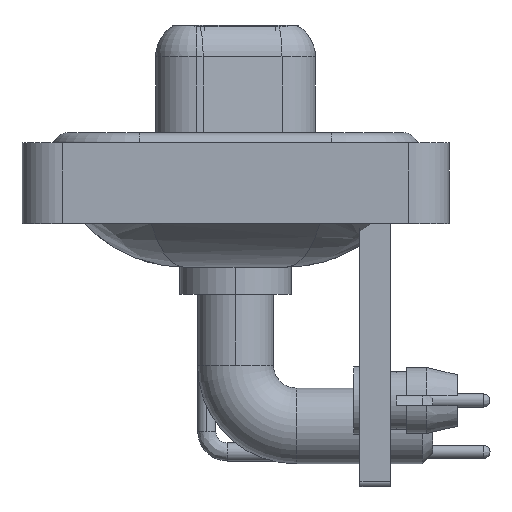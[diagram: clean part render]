
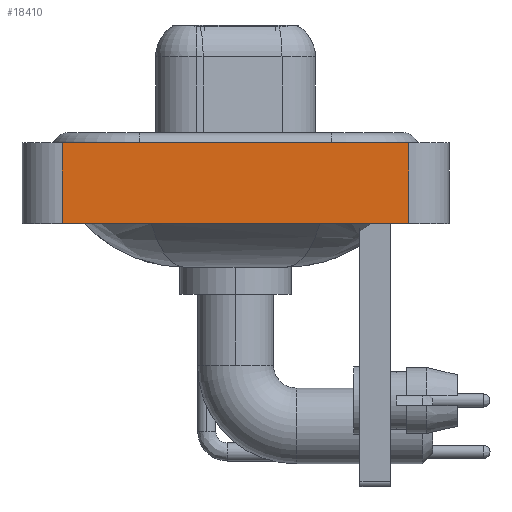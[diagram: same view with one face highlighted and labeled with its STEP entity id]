
A CAD part, left-side view. The second image highlights one B-rep face of the part: STEP entity #18410.
In plain terms, the highlighted planar face has unit normal (-1, 0, 0).
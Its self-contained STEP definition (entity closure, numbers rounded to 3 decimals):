
#1458 = EDGE_CURVE ( 'NONE', #16664, #22199, #5912, .T. ) ;
#3110 = CARTESIAN_POINT ( 'NONE',  ( -7.35, 8.55, -3.6 ) ) ;
#3141 = CARTESIAN_POINT ( 'NONE',  ( -7.35, 8.55, 0.4 ) ) ;
#4253 = CARTESIAN_POINT ( 'NONE',  ( -7.35, -8.55, -3.6 ) ) ;
#4636 = DIRECTION ( 'NONE',  ( 0., 0., 1. ) ) ;
#4999 = ORIENTED_EDGE ( 'NONE', *, *, #1458, .T. ) ;
#5130 = CARTESIAN_POINT ( 'NONE',  ( -7.35, -8.55, -3.6 ) ) ;
#5541 = VECTOR ( 'NONE', #20622, 1000. ) ;
#5754 = CARTESIAN_POINT ( 'NONE',  ( -7.35, -8.55, -3.6 ) ) ;
#5912 = LINE ( 'NONE', #4253, #5541 ) ;
#7413 = ORIENTED_EDGE ( 'NONE', *, *, #11222, .T. ) ;
#7747 = CARTESIAN_POINT ( 'NONE',  ( -7.35, -8.55, 0.4 ) ) ;
#8289 = VERTEX_POINT ( 'NONE', #3141 ) ;
#9542 = DIRECTION ( 'NONE',  ( 0., -1., 0. ) ) ;
#9745 = CARTESIAN_POINT ( 'NONE',  ( -7.35, -8.55, -3.6 ) ) ;
#9794 = VECTOR ( 'NONE', #4636, 1000. ) ;
#11210 = LINE ( 'NONE', #5754, #15427 ) ;
#11222 = EDGE_CURVE ( 'NONE', #15748, #16664, #11210, .T. ) ;
#11332 = DIRECTION ( 'NONE',  ( 0., -1., 0. ) ) ;
#11447 = LINE ( 'NONE', #7747, #13368 ) ;
#11981 = PLANE ( 'NONE',  #17991 ) ;
#13368 = VECTOR ( 'NONE', #11332, 1000. ) ;
#14828 = ORIENTED_EDGE ( 'NONE', *, *, #23007, .F. ) ;
#15054 = EDGE_CURVE ( 'NONE', #8289, #22199, #11447, .T. ) ;
#15427 = VECTOR ( 'NONE', #9542, 1000. ) ;
#15748 = VERTEX_POINT ( 'NONE', #18052 ) ;
#16390 = ORIENTED_EDGE ( 'NONE', *, *, #15054, .F. ) ;
#16664 = VERTEX_POINT ( 'NONE', #5130 ) ;
#17991 = AXIS2_PLACEMENT_3D ( 'NONE', #9745, #20656, #18870 ) ;
#18052 = CARTESIAN_POINT ( 'NONE',  ( -7.35, 8.55, -3.6 ) ) ;
#18364 = CARTESIAN_POINT ( 'NONE',  ( -7.35, -8.55, 0.4 ) ) ;
#18410 = ADVANCED_FACE ( 'NONE', ( #19227 ), #11981, .T. ) ;
#18870 = DIRECTION ( 'NONE',  ( 0., 0., 1. ) ) ;
#19227 = FACE_OUTER_BOUND ( 'NONE', #21508, .T. ) ;
#20622 = DIRECTION ( 'NONE',  ( 0., 0., 1. ) ) ;
#20656 = DIRECTION ( 'NONE',  ( -1., 0., 0. ) ) ;
#21508 = EDGE_LOOP ( 'NONE', ( #4999, #16390, #14828, #7413 ) ) ;
#22199 = VERTEX_POINT ( 'NONE', #18364 ) ;
#23007 = EDGE_CURVE ( 'NONE', #15748, #8289, #23158, .T. ) ;
#23158 = LINE ( 'NONE', #3110, #9794 ) ;
